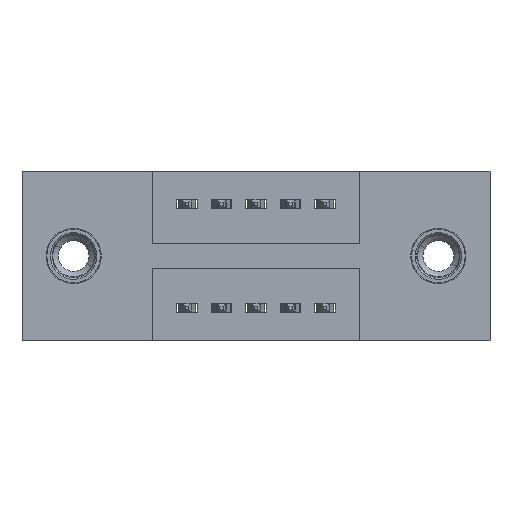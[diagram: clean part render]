
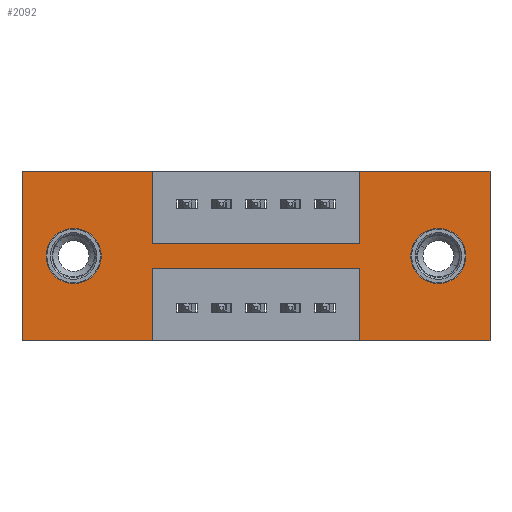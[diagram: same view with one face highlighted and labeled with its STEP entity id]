
A CAD part, front view. The second image highlights one B-rep face of the part: STEP entity #2092.
In plain terms, the highlighted planar face has unit normal (0, -1, 0).
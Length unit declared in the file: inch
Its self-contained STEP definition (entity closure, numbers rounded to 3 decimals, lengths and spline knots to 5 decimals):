
#92 = FACE_OUTER_BOUND ( 'NONE', #3965, .T. ) ;
#96 = EDGE_CURVE ( 'NONE', #8260, #1330, #6942, .T. ) ;
#104 = LINE ( 'NONE', #4934, #2109 ) ;
#165 = CARTESIAN_POINT ( 'NONE',  ( 0., 0., 0. ) ) ;
#178 = ORIENTED_EDGE ( 'NONE', *, *, #8971, .T. ) ;
#199 = DIRECTION ( 'NONE',  ( 0., 0., 1. ) ) ;
#239 = CARTESIAN_POINT ( 'NONE',  ( 0.9775, 0., 0. ) ) ;
#249 = VERTEX_POINT ( 'NONE', #3492 ) ;
#338 = EDGE_CURVE ( 'NONE', #603, #8260, #4713, .T. ) ;
#516 = VECTOR ( 'NONE', #8762, 39.37008 ) ;
#596 = DIRECTION ( 'NONE',  ( 0., 0., 1. ) ) ;
#603 = VERTEX_POINT ( 'NONE', #3126 ) ;
#655 = CARTESIAN_POINT ( 'NONE',  ( 0.3775, 0., -0.21 ) ) ;
#677 = LINE ( 'NONE', #3339, #3579 ) ;
#861 = ORIENTED_EDGE ( 'NONE', *, *, #1601, .F. ) ;
#928 = DIRECTION ( 'NONE',  ( 1., 0., 0. ) ) ;
#1040 = CARTESIAN_POINT ( 'NONE',  ( 1.2055, 0., -0.165 ) ) ;
#1076 = DIRECTION ( 'NONE',  ( 0., 0., -1. ) ) ;
#1164 = VERTEX_POINT ( 'NONE', #6793 ) ;
#1230 = LINE ( 'NONE', #4851, #5479 ) ;
#1330 = VERTEX_POINT ( 'NONE', #3513 ) ;
#1503 = CARTESIAN_POINT ( 'NONE',  ( 0.1495, 0., -0.325 ) ) ;
#1601 = EDGE_CURVE ( 'NONE', #1330, #6305, #104, .T. ) ;
#1657 = AXIS2_PLACEMENT_3D ( 'NONE', #6790, #5239, #3968 ) ;
#1734 = DIRECTION ( 'NONE',  ( 0., 1., 0. ) ) ;
#1831 = EDGE_CURVE ( 'NONE', #4995, #603, #7236, .T. ) ;
#1846 = EDGE_CURVE ( 'NONE', #4983, #8923, #6586, .T. ) ;
#1853 = CARTESIAN_POINT ( 'NONE',  ( 0.9775, 0., -0.28 ) ) ;
#1976 = VERTEX_POINT ( 'NONE', #7426 ) ;
#2002 = EDGE_LOOP ( 'NONE', ( #4509, #3604 ) ) ;
#2078 = LINE ( 'NONE', #3794, #516 ) ;
#2088 = AXIS2_PLACEMENT_3D ( 'NONE', #8401, #4148, #596 ) ;
#2091 = DIRECTION ( 'NONE',  ( 0., 0., 1. ) ) ;
#2092 = ADVANCED_FACE ( 'NONE', ( #2785, #2896, #92 ), #4350, .T. ) ;
#2109 = VECTOR ( 'NONE', #2091, 39.37008 ) ;
#2136 = VERTEX_POINT ( 'NONE', #1040 ) ;
#2454 = CARTESIAN_POINT ( 'NONE',  ( 0.1495, 0., -0.245 ) ) ;
#2489 = CARTESIAN_POINT ( 'NONE',  ( 0.9775, 0., -0.28 ) ) ;
#2617 = VECTOR ( 'NONE', #8620, 39.37008 ) ;
#2768 = ORIENTED_EDGE ( 'NONE', *, *, #1831, .F. ) ;
#2785 = FACE_BOUND ( 'NONE', #2002, .T. ) ;
#2896 = FACE_BOUND ( 'NONE', #4007, .T. ) ;
#2918 = VECTOR ( 'NONE', #3189, 39.37008 ) ;
#2936 = EDGE_CURVE ( 'NONE', #5217, #4968, #9108, .T. ) ;
#2976 = ORIENTED_EDGE ( 'NONE', *, *, #7764, .F. ) ;
#2998 = ORIENTED_EDGE ( 'NONE', *, *, #3768, .F. ) ;
#3035 = ORIENTED_EDGE ( 'NONE', *, *, #338, .F. ) ;
#3099 = AXIS2_PLACEMENT_3D ( 'NONE', #3817, #6678, #6006 ) ;
#3126 = CARTESIAN_POINT ( 'NONE',  ( 0.3775, 0., -0.28 ) ) ;
#3141 = CARTESIAN_POINT ( 'NONE',  ( 1.355, 0., -0.49 ) ) ;
#3144 = VERTEX_POINT ( 'NONE', #3310 ) ;
#3189 = DIRECTION ( 'NONE',  ( -1., 0., 0. ) ) ;
#3310 = CARTESIAN_POINT ( 'NONE',  ( 1.2055, 0., -0.325 ) ) ;
#3338 = LINE ( 'NONE', #1853, #8547 ) ;
#3339 = CARTESIAN_POINT ( 'NONE',  ( 0., 0., -0.49 ) ) ;
#3478 = VECTOR ( 'NONE', #5647, 39.37008 ) ;
#3492 = CARTESIAN_POINT ( 'NONE',  ( 0.3775, 0., -0.21 ) ) ;
#3513 = CARTESIAN_POINT ( 'NONE',  ( 0., 0., -0.49 ) ) ;
#3531 = VERTEX_POINT ( 'NONE', #9099 ) ;
#3579 = VECTOR ( 'NONE', #4800, 39.37008 ) ;
#3596 = ORIENTED_EDGE ( 'NONE', *, *, #2936, .T. ) ;
#3604 = ORIENTED_EDGE ( 'NONE', *, *, #3975, .T. ) ;
#3768 = EDGE_CURVE ( 'NONE', #249, #1164, #2078, .T. ) ;
#3794 = CARTESIAN_POINT ( 'NONE',  ( 0.3775, 0., -0.21 ) ) ;
#3817 = CARTESIAN_POINT ( 'NONE',  ( 0., 0., -0.49 ) ) ;
#3965 = EDGE_LOOP ( 'NONE', ( #5615, #2998, #9058, #6194, #861, #4177, #3035, #2768, #2976, #7148, #7991, #6470 ) ) ;
#3968 = DIRECTION ( 'NONE',  ( 0., 0., -1. ) ) ;
#3975 = EDGE_CURVE ( 'NONE', #3144, #2136, #7532, .T. ) ;
#4007 = EDGE_LOOP ( 'NONE', ( #178, #3596 ) ) ;
#4134 = VECTOR ( 'NONE', #928, 39.37008 ) ;
#4148 = DIRECTION ( 'NONE',  ( 0., 1., 0. ) ) ;
#4177 = ORIENTED_EDGE ( 'NONE', *, *, #96, .F. ) ;
#4295 = LINE ( 'NONE', #7959, #2617 ) ;
#4350 = PLANE ( 'NONE',  #3099 ) ;
#4509 = ORIENTED_EDGE ( 'NONE', *, *, #5055, .T. ) ;
#4626 = CARTESIAN_POINT ( 'NONE',  ( 0., 0., -0.49 ) ) ;
#4680 = CARTESIAN_POINT ( 'NONE',  ( 0.9775, 0., -0.21 ) ) ;
#4713 = LINE ( 'NONE', #8947, #8031 ) ;
#4786 = EDGE_CURVE ( 'NONE', #8923, #9040, #4295, .T. ) ;
#4800 = DIRECTION ( 'NONE',  ( -1., 0., 0. ) ) ;
#4851 = CARTESIAN_POINT ( 'NONE',  ( 0., 0., 0. ) ) ;
#4934 = CARTESIAN_POINT ( 'NONE',  ( 0., 0., 0. ) ) ;
#4957 = CARTESIAN_POINT ( 'NONE',  ( 1.2055, 0., -0.245 ) ) ;
#4968 = VERTEX_POINT ( 'NONE', #6026 ) ;
#4983 = VERTEX_POINT ( 'NONE', #239 ) ;
#4995 = VERTEX_POINT ( 'NONE', #2489 ) ;
#5055 = EDGE_CURVE ( 'NONE', #2136, #3144, #6528, .T. ) ;
#5172 = DIRECTION ( 'NONE',  ( 0., 1., 0. ) ) ;
#5194 = DIRECTION ( 'NONE',  ( -1., 0., 0. ) ) ;
#5217 = VERTEX_POINT ( 'NONE', #1503 ) ;
#5239 = DIRECTION ( 'NONE',  ( 0., 1., 0. ) ) ;
#5256 = EDGE_CURVE ( 'NONE', #1164, #4983, #5460, .T. ) ;
#5276 = CARTESIAN_POINT ( 'NONE',  ( 0.3775, 0., -0.49 ) ) ;
#5460 = LINE ( 'NONE', #4680, #5997 ) ;
#5479 = VECTOR ( 'NONE', #8386, 39.37008 ) ;
#5615 = ORIENTED_EDGE ( 'NONE', *, *, #5256, .F. ) ;
#5647 = DIRECTION ( 'NONE',  ( 0., 0., -1. ) ) ;
#5712 = AXIS2_PLACEMENT_3D ( 'NONE', #2454, #5172, #199 ) ;
#5826 = CARTESIAN_POINT ( 'NONE',  ( 0., 0., 0. ) ) ;
#5997 = VECTOR ( 'NONE', #8212, 39.37008 ) ;
#6002 = EDGE_CURVE ( 'NONE', #9040, #3531, #677, .T. ) ;
#6006 = DIRECTION ( 'NONE',  ( 0., 0., -1. ) ) ;
#6026 = CARTESIAN_POINT ( 'NONE',  ( 0.1495, 0., -0.165 ) ) ;
#6170 = EDGE_CURVE ( 'NONE', #1976, #249, #7341, .T. ) ;
#6194 = ORIENTED_EDGE ( 'NONE', *, *, #6650, .F. ) ;
#6305 = VERTEX_POINT ( 'NONE', #5826 ) ;
#6470 = ORIENTED_EDGE ( 'NONE', *, *, #1846, .F. ) ;
#6528 = CIRCLE ( 'NONE', #1657, 0.08 ) ;
#6586 = LINE ( 'NONE', #165, #4134 ) ;
#6650 = EDGE_CURVE ( 'NONE', #6305, #1976, #1230, .T. ) ;
#6678 = DIRECTION ( 'NONE',  ( 0., -1., 0. ) ) ;
#6790 = CARTESIAN_POINT ( 'NONE',  ( 1.2055, 0., -0.245 ) ) ;
#6793 = CARTESIAN_POINT ( 'NONE',  ( 0.9775, 0., -0.21 ) ) ;
#6907 = DIRECTION ( 'NONE',  ( 0., 0., -1. ) ) ;
#6942 = LINE ( 'NONE', #4626, #2918 ) ;
#7148 = ORIENTED_EDGE ( 'NONE', *, *, #6002, .F. ) ;
#7236 = LINE ( 'NONE', #7396, #8904 ) ;
#7284 = CARTESIAN_POINT ( 'NONE',  ( 1.355, 0., 0. ) ) ;
#7341 = LINE ( 'NONE', #655, #3478 ) ;
#7396 = CARTESIAN_POINT ( 'NONE',  ( 0.3775, 0., -0.28 ) ) ;
#7426 = CARTESIAN_POINT ( 'NONE',  ( 0.3775, 0., 0. ) ) ;
#7532 = CIRCLE ( 'NONE', #8710, 0.08 ) ;
#7764 = EDGE_CURVE ( 'NONE', #3531, #4995, #3338, .T. ) ;
#7959 = CARTESIAN_POINT ( 'NONE',  ( 1.355, 0., 0. ) ) ;
#7991 = ORIENTED_EDGE ( 'NONE', *, *, #4786, .F. ) ;
#8031 = VECTOR ( 'NONE', #6907, 39.37008 ) ;
#8041 = DIRECTION ( 'NONE',  ( 0., 0., 1. ) ) ;
#8212 = DIRECTION ( 'NONE',  ( 0., 0., 1. ) ) ;
#8260 = VERTEX_POINT ( 'NONE', #5276 ) ;
#8386 = DIRECTION ( 'NONE',  ( 1., 0., 0. ) ) ;
#8401 = CARTESIAN_POINT ( 'NONE',  ( 0.1495, 0., -0.245 ) ) ;
#8547 = VECTOR ( 'NONE', #8041, 39.37008 ) ;
#8620 = DIRECTION ( 'NONE',  ( 0., 0., -1. ) ) ;
#8710 = AXIS2_PLACEMENT_3D ( 'NONE', #4957, #1734, #1076 ) ;
#8762 = DIRECTION ( 'NONE',  ( 1., 0., 0. ) ) ;
#8904 = VECTOR ( 'NONE', #5194, 39.37008 ) ;
#8923 = VERTEX_POINT ( 'NONE', #7284 ) ;
#8947 = CARTESIAN_POINT ( 'NONE',  ( 0.3775, 0., -0.28 ) ) ;
#8971 = EDGE_CURVE ( 'NONE', #4968, #5217, #9197, .T. ) ;
#9040 = VERTEX_POINT ( 'NONE', #3141 ) ;
#9058 = ORIENTED_EDGE ( 'NONE', *, *, #6170, .F. ) ;
#9099 = CARTESIAN_POINT ( 'NONE',  ( 0.9775, 0., -0.49 ) ) ;
#9108 = CIRCLE ( 'NONE', #2088, 0.08 ) ;
#9197 = CIRCLE ( 'NONE', #5712, 0.08 ) ;
